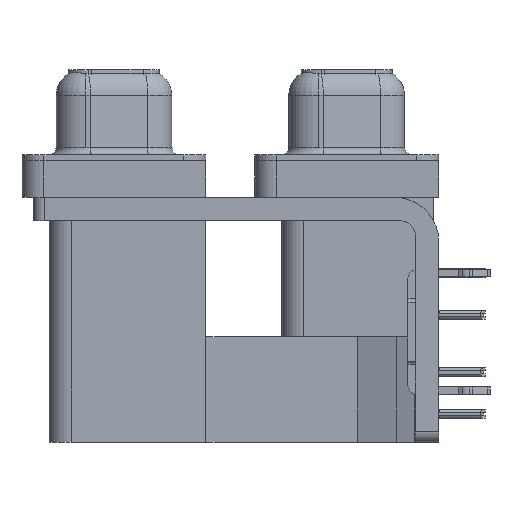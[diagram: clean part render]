
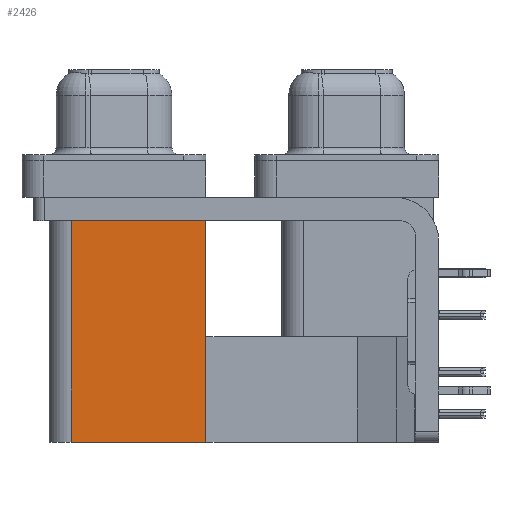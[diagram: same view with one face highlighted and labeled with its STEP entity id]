
A CAD part, left-side view. The second image highlights one B-rep face of the part: STEP entity #2426.
In plain terms, the highlighted planar face has unit normal (-1, 0, 0).
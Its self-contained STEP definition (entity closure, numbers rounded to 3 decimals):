
#649 = DIRECTION ( 'NONE',  ( 0., 0., 1. ) ) ;
#2426 = ADVANCED_FACE ( 'NONE', ( #24089 ), #33532, .F. ) ;
#4661 = DIRECTION ( 'NONE',  ( 0., 1., 0. ) ) ;
#6818 = CARTESIAN_POINT ( 'NONE',  ( 3.79, 18.8, -19.2 ) ) ;
#7854 = CARTESIAN_POINT ( 'NONE',  ( 3.79, 9.6, -19.2 ) ) ;
#7957 = CARTESIAN_POINT ( 'NONE',  ( 3.79, 18.8, -2.5 ) ) ;
#9514 = CARTESIAN_POINT ( 'NONE',  ( 3.79, 9.6, -2.5 ) ) ;
#9814 = VERTEX_POINT ( 'NONE', #15970 ) ;
#11170 = VECTOR ( 'NONE', #29967, 1000. ) ;
#11528 = VERTEX_POINT ( 'NONE', #9514 ) ;
#11916 = VERTEX_POINT ( 'NONE', #34844 ) ;
#12490 = EDGE_CURVE ( 'NONE', #9814, #11916, #25987, .T. ) ;
#15392 = EDGE_CURVE ( 'NONE', #11528, #17985, #40526, .T. ) ;
#15843 = LINE ( 'NONE', #19904, #11170 ) ;
#15970 = CARTESIAN_POINT ( 'NONE',  ( 3.79, 9.6, -19.2 ) ) ;
#17447 = AXIS2_PLACEMENT_3D ( 'NONE', #7854, #20909, #4661 ) ;
#17985 = VERTEX_POINT ( 'NONE', #7957 ) ;
#19375 = CARTESIAN_POINT ( 'NONE',  ( 3.79, 9.6, -19.2 ) ) ;
#19672 = ORIENTED_EDGE ( 'NONE', *, *, #12490, .F. ) ;
#19904 = CARTESIAN_POINT ( 'NONE',  ( 3.79, 9.6, -19.2 ) ) ;
#20682 = EDGE_CURVE ( 'NONE', #9814, #11528, #15843, .T. ) ;
#20690 = ORIENTED_EDGE ( 'NONE', *, *, #15392, .T. ) ;
#20909 = DIRECTION ( 'NONE',  ( 1., 0., 0. ) ) ;
#23492 = LINE ( 'NONE', #6818, #41308 ) ;
#24089 = FACE_OUTER_BOUND ( 'NONE', #38931, .T. ) ;
#25126 = EDGE_CURVE ( 'NONE', #11916, #17985, #23492, .T. ) ;
#25987 = LINE ( 'NONE', #19375, #37831 ) ;
#29967 = DIRECTION ( 'NONE',  ( 0., 0., 1. ) ) ;
#30291 = ORIENTED_EDGE ( 'NONE', *, *, #20682, .T. ) ;
#33071 = VECTOR ( 'NONE', #34554, 1000. ) ;
#33532 = PLANE ( 'NONE',  #17447 ) ;
#34554 = DIRECTION ( 'NONE',  ( 0., 1., 0. ) ) ;
#34844 = CARTESIAN_POINT ( 'NONE',  ( 3.79, 18.8, -19.2 ) ) ;
#37118 = CARTESIAN_POINT ( 'NONE',  ( 3.79, 9.6, -2.5 ) ) ;
#37831 = VECTOR ( 'NONE', #38193, 1000. ) ;
#38193 = DIRECTION ( 'NONE',  ( 0., 1., 0. ) ) ;
#38602 = ORIENTED_EDGE ( 'NONE', *, *, #25126, .F. ) ;
#38931 = EDGE_LOOP ( 'NONE', ( #20690, #38602, #19672, #30291 ) ) ;
#40526 = LINE ( 'NONE', #37118, #33071 ) ;
#41308 = VECTOR ( 'NONE', #649, 1000. ) ;
